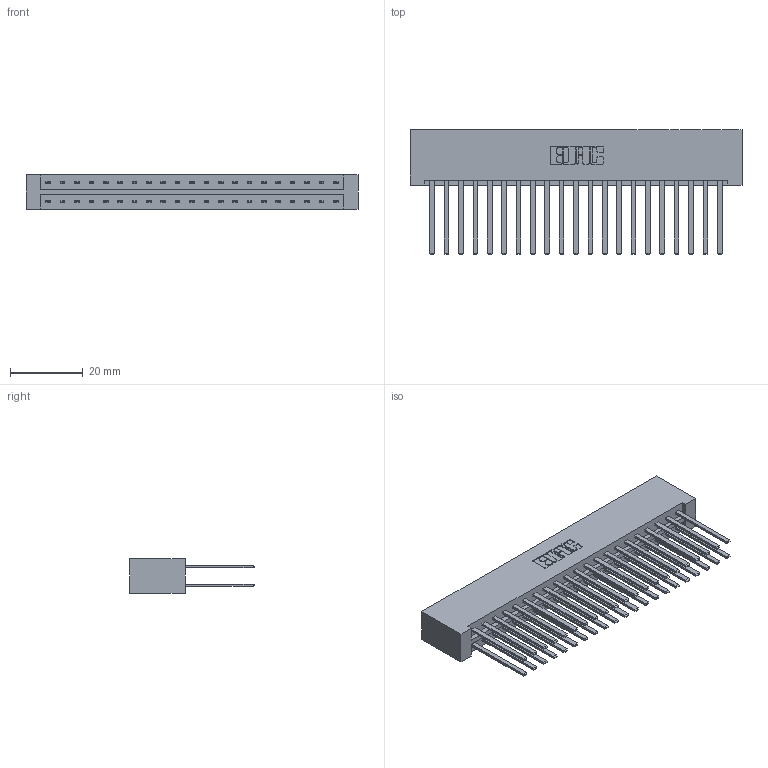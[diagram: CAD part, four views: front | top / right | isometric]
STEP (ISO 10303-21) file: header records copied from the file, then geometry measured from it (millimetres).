
FILE_DESCRIPTION (( 'STEP AP203' ), '1' );
FILE_NAME ('333-042-544-201.STEP', '2018-08-03T19:14:48', ( '' ), ( '' ), 'SwSTEP 2.0', 'SolidWorks 2016', '' );
FILE_SCHEMA (( 'CONFIG_CONTROL_DESIGN' ));
Length unit declared in the file: inch
Products named in the file (3): 333 Part_Lugless; 345-292-001_345-293-144; 333-042-544-201
Assembly tree (43 placements, depth 2):
  333-042-544-201
    333 Part_Lugless
    345-292-001_345-293-144  x42
Bounding box: 91.47 x 34.3 x 9.4 mm (x, y, z)
Volume: 10362.7 mm3; surface area: 13945.7 mm2
Topology: 43 solids, 43 shells, 2038 faces, 6041 edges, 3970 vertices
Faces by surface type: plane 1410, cylinder 628
Entity records: 15765 total; most frequent: CARTESIAN_POINT 2634, ORIENTED_EDGE 2570, DIRECTION 2277, EDGE_CURVE 1285, VECTOR 1169, LINE 1169, VERTEX_POINT 854, AXIS2_PLACEMENT_3D 554
